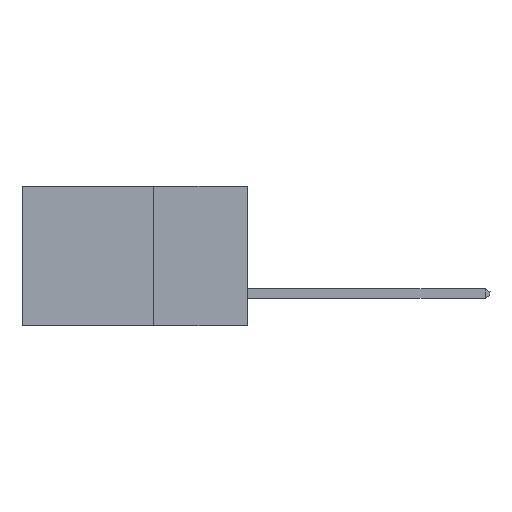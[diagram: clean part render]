
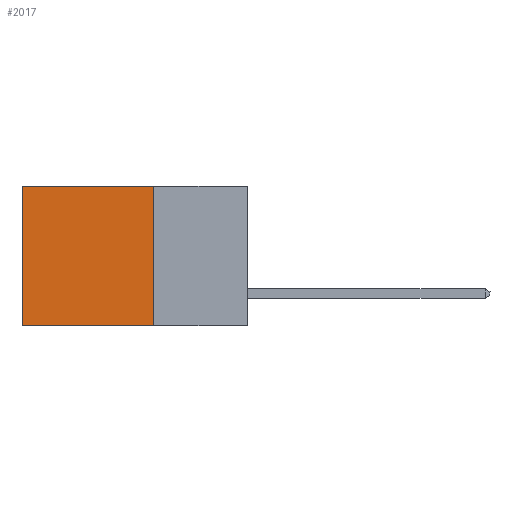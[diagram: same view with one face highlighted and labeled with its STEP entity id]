
A CAD part, left-side view. The second image highlights one B-rep face of the part: STEP entity #2017.
In plain terms, the highlighted planar face has unit normal (-1, 0, 0).
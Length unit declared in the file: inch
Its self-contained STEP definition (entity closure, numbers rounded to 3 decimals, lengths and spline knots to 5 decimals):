
#697 = ORIENTED_EDGE ( 'NONE', *, *, #3964, .T. ) ;
#1535 = CARTESIAN_POINT ( 'NONE',  ( 0.2615, 0.25, -0.37 ) ) ;
#1757 = DIRECTION ( 'NONE',  ( 0., 0., -1. ) ) ;
#1810 = CARTESIAN_POINT ( 'NONE',  ( 0.2615, 0.25, 0. ) ) ;
#2017 = ADVANCED_FACE ( 'NONE', ( #7188 ), #4906, .F. ) ;
#2069 = DIRECTION ( 'NONE',  ( 0., 0., -1. ) ) ;
#2127 = ORIENTED_EDGE ( 'NONE', *, *, #2615, .T. ) ;
#2615 = EDGE_CURVE ( 'NONE', #7053, #4835, #8118, .T. ) ;
#2713 = EDGE_CURVE ( 'NONE', #10025, #3627, #5401, .T. ) ;
#3627 = VERTEX_POINT ( 'NONE', #6305 ) ;
#3908 = DIRECTION ( 'NONE',  ( 1., 0., 0. ) ) ;
#3964 = EDGE_CURVE ( 'NONE', #4835, #3627, #9221, .T. ) ;
#4180 = VECTOR ( 'NONE', #6805, 39.37008 ) ;
#4467 = ORIENTED_EDGE ( 'NONE', *, *, #6275, .F. ) ;
#4504 = VECTOR ( 'NONE', #2069, 39.37008 ) ;
#4835 = VERTEX_POINT ( 'NONE', #8156 ) ;
#4906 = PLANE ( 'NONE',  #9677 ) ;
#5048 = LINE ( 'NONE', #9890, #5490 ) ;
#5401 = LINE ( 'NONE', #1535, #8627 ) ;
#5490 = VECTOR ( 'NONE', #1757, 39.37008 ) ;
#5531 = CARTESIAN_POINT ( 'NONE',  ( 0.2615, 0.25, -0.37 ) ) ;
#5780 = CARTESIAN_POINT ( 'NONE',  ( 0.2615, 0.25, 0. ) ) ;
#6275 = EDGE_CURVE ( 'NONE', #7053, #10025, #5048, .T. ) ;
#6305 = CARTESIAN_POINT ( 'NONE',  ( 0.2615, 0.6, -0.37 ) ) ;
#6805 = DIRECTION ( 'NONE',  ( 0., 1., 0. ) ) ;
#7053 = VERTEX_POINT ( 'NONE', #5780 ) ;
#7188 = FACE_OUTER_BOUND ( 'NONE', #10079, .T. ) ;
#7593 = CARTESIAN_POINT ( 'NONE',  ( 0.2615, 0.25, -0.37 ) ) ;
#7606 = ORIENTED_EDGE ( 'NONE', *, *, #2713, .F. ) ;
#7736 = DIRECTION ( 'NONE',  ( 0., 1., 0. ) ) ;
#8118 = LINE ( 'NONE', #1810, #4180 ) ;
#8156 = CARTESIAN_POINT ( 'NONE',  ( 0.2615, 0.6, 0. ) ) ;
#8627 = VECTOR ( 'NONE', #7736, 39.37008 ) ;
#8868 = DIRECTION ( 'NONE',  ( 0., 0., -1. ) ) ;
#9221 = LINE ( 'NONE', #10055, #4504 ) ;
#9677 = AXIS2_PLACEMENT_3D ( 'NONE', #5531, #3908, #8868 ) ;
#9890 = CARTESIAN_POINT ( 'NONE',  ( 0.2615, 0.25, -0.37 ) ) ;
#10025 = VERTEX_POINT ( 'NONE', #7593 ) ;
#10055 = CARTESIAN_POINT ( 'NONE',  ( 0.2615, 0.6, -0.37 ) ) ;
#10079 = EDGE_LOOP ( 'NONE', ( #697, #7606, #4467, #2127 ) ) ;
